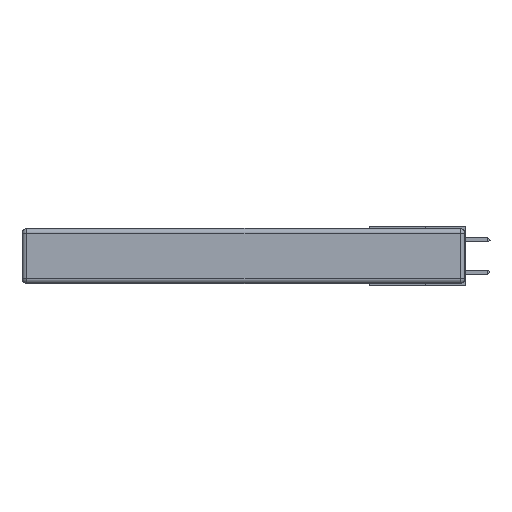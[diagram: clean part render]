
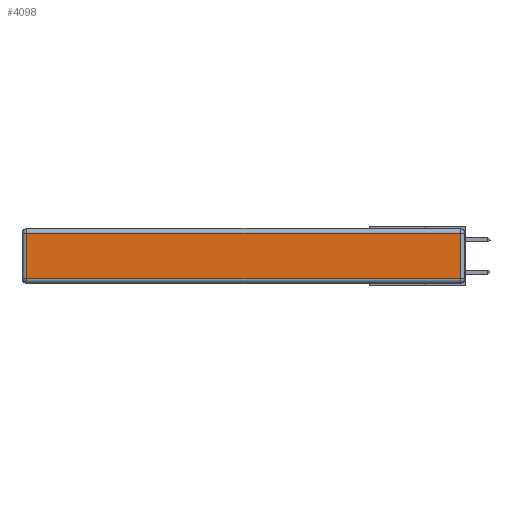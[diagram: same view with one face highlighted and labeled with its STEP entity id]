
A CAD part, left-side view. The second image highlights one B-rep face of the part: STEP entity #4098.
In plain terms, the highlighted planar face has unit normal (-1, 0, 0).
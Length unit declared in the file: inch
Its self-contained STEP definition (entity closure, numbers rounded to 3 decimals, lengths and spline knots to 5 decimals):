
#272 = CARTESIAN_POINT ( 'NONE',  ( 0., 0.03, -0.343 ) ) ;
#3805 = AXIS2_PLACEMENT_3D ( 'NONE', #13545, #22191, #22436 ) ;
#4098 = ADVANCED_FACE ( 'NONE', ( #7721 ), #32623, .T. ) ;
#4468 = CARTESIAN_POINT ( 'NONE',  ( 0., 2.75, -0.03 ) ) ;
#5304 = DIRECTION ( 'NONE',  ( 0., 0., -1. ) ) ;
#5337 = CARTESIAN_POINT ( 'NONE',  ( 0., 0.03, -0.03 ) ) ;
#5498 = LINE ( 'NONE', #272, #22650 ) ;
#5804 = DIRECTION ( 'NONE',  ( 0., 0., 1. ) ) ;
#6763 = VERTEX_POINT ( 'NONE', #26883 ) ;
#7553 = EDGE_LOOP ( 'NONE', ( #10659, #30286, #11185, #25529 ) ) ;
#7677 = EDGE_CURVE ( 'NONE', #20550, #19628, #21924, .T. ) ;
#7721 = FACE_OUTER_BOUND ( 'NONE', #7553, .T. ) ;
#8027 = LINE ( 'NONE', #32102, #21804 ) ;
#10659 = ORIENTED_EDGE ( 'NONE', *, *, #7677, .T. ) ;
#11185 = ORIENTED_EDGE ( 'NONE', *, *, #14417, .T. ) ;
#12969 = DIRECTION ( 'NONE',  ( 0., 1., 0. ) ) ;
#13545 = CARTESIAN_POINT ( 'NONE',  ( 0., 0., -0.343 ) ) ;
#14417 = EDGE_CURVE ( 'NONE', #19593, #6763, #28690, .T. ) ;
#16073 = CARTESIAN_POINT ( 'NONE',  ( 0., 0.03, -0.313 ) ) ;
#16168 = CARTESIAN_POINT ( 'NONE',  ( 0., 2.72, -0.313 ) ) ;
#19593 = VERTEX_POINT ( 'NONE', #5337 ) ;
#19628 = VERTEX_POINT ( 'NONE', #16073 ) ;
#20550 = VERTEX_POINT ( 'NONE', #16168 ) ;
#21804 = VECTOR ( 'NONE', #5304, 39.37008 ) ;
#21924 = LINE ( 'NONE', #28802, #23994 ) ;
#21976 = VECTOR ( 'NONE', #12969, 39.37008 ) ;
#22191 = DIRECTION ( 'NONE',  ( -1., 0., 0. ) ) ;
#22436 = DIRECTION ( 'NONE',  ( 0., 0., 1. ) ) ;
#22650 = VECTOR ( 'NONE', #5804, 39.37008 ) ;
#23994 = VECTOR ( 'NONE', #28467, 39.37008 ) ;
#25529 = ORIENTED_EDGE ( 'NONE', *, *, #32188, .T. ) ;
#26883 = CARTESIAN_POINT ( 'NONE',  ( 0., 2.72, -0.03 ) ) ;
#28467 = DIRECTION ( 'NONE',  ( 0., -1., 0. ) ) ;
#28690 = LINE ( 'NONE', #4468, #21976 ) ;
#28802 = CARTESIAN_POINT ( 'NONE',  ( 0., 0., -0.313 ) ) ;
#30286 = ORIENTED_EDGE ( 'NONE', *, *, #31923, .T. ) ;
#31923 = EDGE_CURVE ( 'NONE', #19628, #19593, #5498, .T. ) ;
#32102 = CARTESIAN_POINT ( 'NONE',  ( 0., 2.72, -0.343 ) ) ;
#32188 = EDGE_CURVE ( 'NONE', #6763, #20550, #8027, .T. ) ;
#32623 = PLANE ( 'NONE',  #3805 ) ;
